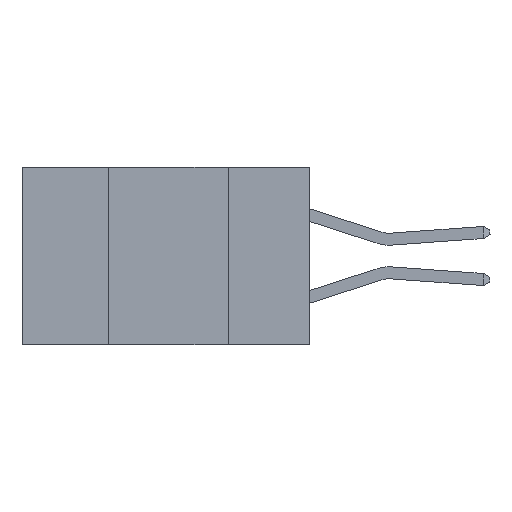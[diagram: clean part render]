
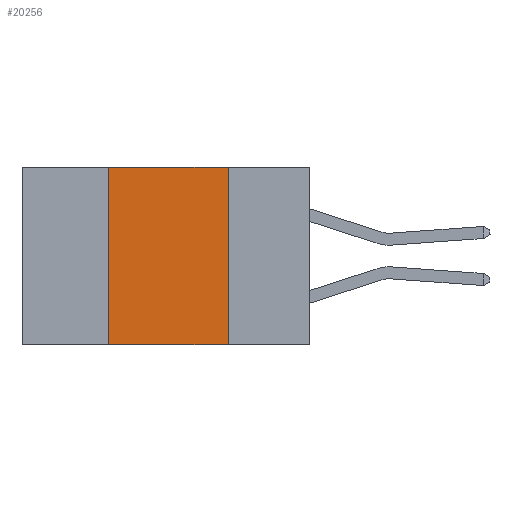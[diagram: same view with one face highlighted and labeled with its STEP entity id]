
A CAD part, left-side view. The second image highlights one B-rep face of the part: STEP entity #20256.
In plain terms, the highlighted planar face has unit normal (-1, 0, 0).
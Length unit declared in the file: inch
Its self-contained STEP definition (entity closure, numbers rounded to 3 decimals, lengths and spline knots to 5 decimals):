
#854 = CARTESIAN_POINT ( 'NONE',  ( 0., 0.17, 0. ) ) ;
#3116 = CARTESIAN_POINT ( 'NONE',  ( 0., 0.6, -0.37 ) ) ;
#4970 = FACE_OUTER_BOUND ( 'NONE', #18366, .T. ) ;
#6019 = CARTESIAN_POINT ( 'NONE',  ( 0., 0.17, 0. ) ) ;
#6135 = CARTESIAN_POINT ( 'NONE',  ( 0., 0.42, 0. ) ) ;
#6320 = PLANE ( 'NONE',  #18395 ) ;
#6709 = VERTEX_POINT ( 'NONE', #10932 ) ;
#8567 = DIRECTION ( 'NONE',  ( 0., 0., -1. ) ) ;
#10342 = LINE ( 'NONE', #21523, #14283 ) ;
#10932 = CARTESIAN_POINT ( 'NONE',  ( 0., 0.17, -0.37 ) ) ;
#13046 = ORIENTED_EDGE ( 'NONE', *, *, #17708, .F. ) ;
#13060 = VECTOR ( 'NONE', #16143, 39.37008 ) ;
#13760 = ORIENTED_EDGE ( 'NONE', *, *, #25161, .T. ) ;
#14283 = VECTOR ( 'NONE', #28005, 39.37008 ) ;
#14501 = EDGE_CURVE ( 'NONE', #24082, #14904, #10342, .T. ) ;
#14904 = VERTEX_POINT ( 'NONE', #6019 ) ;
#16143 = DIRECTION ( 'NONE',  ( 0., 0., 1. ) ) ;
#17655 = ORIENTED_EDGE ( 'NONE', *, *, #19200, .F. ) ;
#17708 = EDGE_CURVE ( 'NONE', #23569, #24082, #24988, .T. ) ;
#18366 = EDGE_LOOP ( 'NONE', ( #17655, #24300, #13046, #13760 ) ) ;
#18395 = AXIS2_PLACEMENT_3D ( 'NONE', #19883, #22114, #8567 ) ;
#18476 = LINE ( 'NONE', #854, #24408 ) ;
#19200 = EDGE_CURVE ( 'NONE', #14904, #6709, #18476, .T. ) ;
#19883 = CARTESIAN_POINT ( 'NONE',  ( 0., 0.6, 0. ) ) ;
#20256 = ADVANCED_FACE ( 'NONE', ( #4970 ), #6320, .F. ) ;
#21198 = DIRECTION ( 'NONE',  ( 0., -1., 0. ) ) ;
#21523 = CARTESIAN_POINT ( 'NONE',  ( 0., 0.6, 0. ) ) ;
#21878 = CARTESIAN_POINT ( 'NONE',  ( 0., 0.42, -0.37 ) ) ;
#22114 = DIRECTION ( 'NONE',  ( 1., 0., 0. ) ) ;
#23331 = DIRECTION ( 'NONE',  ( 0., 0., -1. ) ) ;
#23569 = VERTEX_POINT ( 'NONE', #21878 ) ;
#24082 = VERTEX_POINT ( 'NONE', #6135 ) ;
#24300 = ORIENTED_EDGE ( 'NONE', *, *, #14501, .F. ) ;
#24408 = VECTOR ( 'NONE', #23331, 39.37008 ) ;
#24988 = LINE ( 'NONE', #26031, #13060 ) ;
#25161 = EDGE_CURVE ( 'NONE', #23569, #6709, #28802, .T. ) ;
#26031 = CARTESIAN_POINT ( 'NONE',  ( 0., 0.42, 0. ) ) ;
#28005 = DIRECTION ( 'NONE',  ( 0., -1., 0. ) ) ;
#28130 = VECTOR ( 'NONE', #21198, 39.37008 ) ;
#28802 = LINE ( 'NONE', #3116, #28130 ) ;
